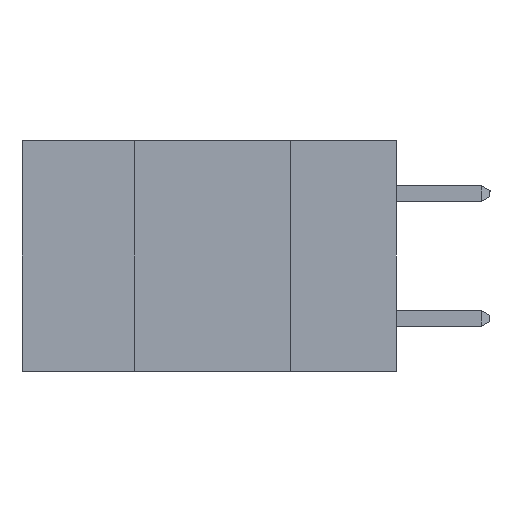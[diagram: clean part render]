
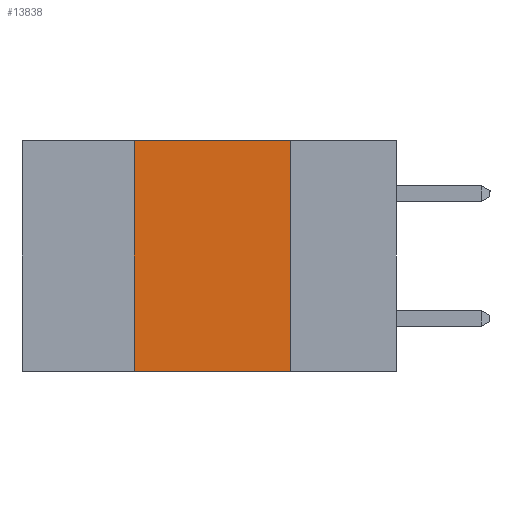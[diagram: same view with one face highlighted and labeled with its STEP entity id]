
A CAD part, left-side view. The second image highlights one B-rep face of the part: STEP entity #13838.
In plain terms, the highlighted planar face has unit normal (-1, 0, 0).
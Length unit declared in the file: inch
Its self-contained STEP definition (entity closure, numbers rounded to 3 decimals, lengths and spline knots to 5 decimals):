
#618 = EDGE_LOOP ( 'NONE', ( #4352, #13392, #19570, #7489 ) ) ;
#762 = VERTEX_POINT ( 'NONE', #21460 ) ;
#830 = DIRECTION ( 'NONE',  ( 1., 0., 0. ) ) ;
#1766 = VECTOR ( 'NONE', #3566, 39.37008 ) ;
#2094 = PLANE ( 'NONE',  #9534 ) ;
#3431 = VERTEX_POINT ( 'NONE', #12231 ) ;
#3566 = DIRECTION ( 'NONE',  ( 0., 0., -1. ) ) ;
#4041 = VERTEX_POINT ( 'NONE', #16677 ) ;
#4352 = ORIENTED_EDGE ( 'NONE', *, *, #8226, .F. ) ;
#5036 = EDGE_CURVE ( 'NONE', #8526, #4041, #12303, .T. ) ;
#6240 = VECTOR ( 'NONE', #20640, 39.37008 ) ;
#6381 = DIRECTION ( 'NONE',  ( 0., 0., 1. ) ) ;
#6512 = DIRECTION ( 'NONE',  ( 0., -1., 0. ) ) ;
#7095 = EDGE_CURVE ( 'NONE', #8526, #762, #18599, .T. ) ;
#7489 = ORIENTED_EDGE ( 'NONE', *, *, #7095, .T. ) ;
#7843 = CARTESIAN_POINT ( 'NONE',  ( 0., 0.6, 0. ) ) ;
#8226 = EDGE_CURVE ( 'NONE', #3431, #762, #10572, .T. ) ;
#8526 = VERTEX_POINT ( 'NONE', #22441 ) ;
#9534 = AXIS2_PLACEMENT_3D ( 'NONE', #7843, #830, #21887 ) ;
#9956 = CARTESIAN_POINT ( 'NONE',  ( 0., 0.6, -0.37 ) ) ;
#10479 = LINE ( 'NONE', #17511, #6240 ) ;
#10572 = LINE ( 'NONE', #21078, #1766 ) ;
#11292 = EDGE_CURVE ( 'NONE', #4041, #3431, #10479, .T. ) ;
#12231 = CARTESIAN_POINT ( 'NONE',  ( 0., 0.17, 0. ) ) ;
#12303 = LINE ( 'NONE', #17610, #17865 ) ;
#13392 = ORIENTED_EDGE ( 'NONE', *, *, #11292, .F. ) ;
#13838 = ADVANCED_FACE ( 'NONE', ( #19704 ), #2094, .F. ) ;
#16677 = CARTESIAN_POINT ( 'NONE',  ( 0., 0.42, 0. ) ) ;
#17511 = CARTESIAN_POINT ( 'NONE',  ( 0., 0.6, 0. ) ) ;
#17539 = VECTOR ( 'NONE', #6512, 39.37008 ) ;
#17610 = CARTESIAN_POINT ( 'NONE',  ( 0., 0.42, -0.37 ) ) ;
#17865 = VECTOR ( 'NONE', #6381, 39.37008 ) ;
#18599 = LINE ( 'NONE', #9956, #17539 ) ;
#19570 = ORIENTED_EDGE ( 'NONE', *, *, #5036, .F. ) ;
#19704 = FACE_OUTER_BOUND ( 'NONE', #618, .T. ) ;
#20640 = DIRECTION ( 'NONE',  ( 0., -1., 0. ) ) ;
#21078 = CARTESIAN_POINT ( 'NONE',  ( 0., 0.17, -0.37 ) ) ;
#21460 = CARTESIAN_POINT ( 'NONE',  ( 0., 0.17, -0.37 ) ) ;
#21887 = DIRECTION ( 'NONE',  ( 0., 0., -1. ) ) ;
#22441 = CARTESIAN_POINT ( 'NONE',  ( 0., 0.42, -0.37 ) ) ;
